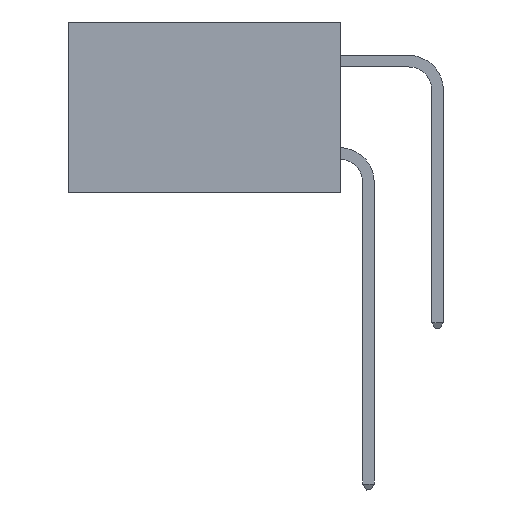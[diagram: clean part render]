
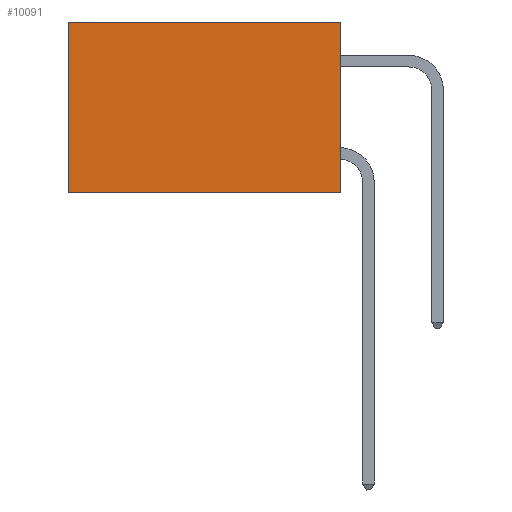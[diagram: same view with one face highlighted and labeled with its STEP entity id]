
A CAD part, left-side view. The second image highlights one B-rep face of the part: STEP entity #10091.
In plain terms, the highlighted planar face has unit normal (-1, 0, 0).
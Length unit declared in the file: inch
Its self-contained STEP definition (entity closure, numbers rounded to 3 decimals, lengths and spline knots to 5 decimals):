
#435 = CARTESIAN_POINT ( 'NONE',  ( 0.277, 0., -0.37 ) ) ;
#1438 = CARTESIAN_POINT ( 'NONE',  ( 0.277, 0.59, 0. ) ) ;
#1603 = ORIENTED_EDGE ( 'NONE', *, *, #16531, .T. ) ;
#2411 = EDGE_LOOP ( 'NONE', ( #1603, #8150, #9509, #8167 ) ) ;
#2507 = LINE ( 'NONE', #14848, #3039 ) ;
#2927 = VERTEX_POINT ( 'NONE', #4982 ) ;
#3039 = VECTOR ( 'NONE', #6343, 39.37008 ) ;
#3418 = DIRECTION ( 'NONE',  ( 0., 1., 0. ) ) ;
#4375 = VERTEX_POINT ( 'NONE', #8392 ) ;
#4982 = CARTESIAN_POINT ( 'NONE',  ( 0.277, 0., 0. ) ) ;
#5746 = VERTEX_POINT ( 'NONE', #1438 ) ;
#6343 = DIRECTION ( 'NONE',  ( 0., 1., 0. ) ) ;
#7234 = EDGE_CURVE ( 'NONE', #2927, #5746, #20018, .T. ) ;
#7396 = DIRECTION ( 'NONE',  ( 1., 0., 0. ) ) ;
#7733 = VECTOR ( 'NONE', #20577, 39.37008 ) ;
#7942 = CARTESIAN_POINT ( 'NONE',  ( 0.277, 0., -0.37 ) ) ;
#8150 = ORIENTED_EDGE ( 'NONE', *, *, #14871, .F. ) ;
#8167 = ORIENTED_EDGE ( 'NONE', *, *, #7234, .T. ) ;
#8392 = CARTESIAN_POINT ( 'NONE',  ( 0.277, 0.59, -0.37 ) ) ;
#8738 = AXIS2_PLACEMENT_3D ( 'NONE', #435, #7396, #19122 ) ;
#9509 = ORIENTED_EDGE ( 'NONE', *, *, #12538, .F. ) ;
#10091 = ADVANCED_FACE ( 'NONE', ( #13956 ), #17488, .F. ) ;
#11739 = DIRECTION ( 'NONE',  ( 0., 0., -1. ) ) ;
#12205 = LINE ( 'NONE', #13966, #7733 ) ;
#12538 = EDGE_CURVE ( 'NONE', #2927, #14802, #16767, .T. ) ;
#13956 = FACE_OUTER_BOUND ( 'NONE', #2411, .T. ) ;
#13966 = CARTESIAN_POINT ( 'NONE',  ( 0.277, 0.59, -0.37 ) ) ;
#14802 = VERTEX_POINT ( 'NONE', #7942 ) ;
#14848 = CARTESIAN_POINT ( 'NONE',  ( 0.277, 0., -0.37 ) ) ;
#14871 = EDGE_CURVE ( 'NONE', #14802, #4375, #2507, .T. ) ;
#15677 = VECTOR ( 'NONE', #3418, 39.37008 ) ;
#16531 = EDGE_CURVE ( 'NONE', #5746, #4375, #12205, .T. ) ;
#16767 = LINE ( 'NONE', #18387, #20546 ) ;
#17488 = PLANE ( 'NONE',  #8738 ) ;
#18387 = CARTESIAN_POINT ( 'NONE',  ( 0.277, 0., -0.37 ) ) ;
#18637 = CARTESIAN_POINT ( 'NONE',  ( 0.277, 0., 0. ) ) ;
#19122 = DIRECTION ( 'NONE',  ( 0., 0., -1. ) ) ;
#20018 = LINE ( 'NONE', #18637, #15677 ) ;
#20546 = VECTOR ( 'NONE', #11739, 39.37008 ) ;
#20577 = DIRECTION ( 'NONE',  ( 0., 0., -1. ) ) ;
